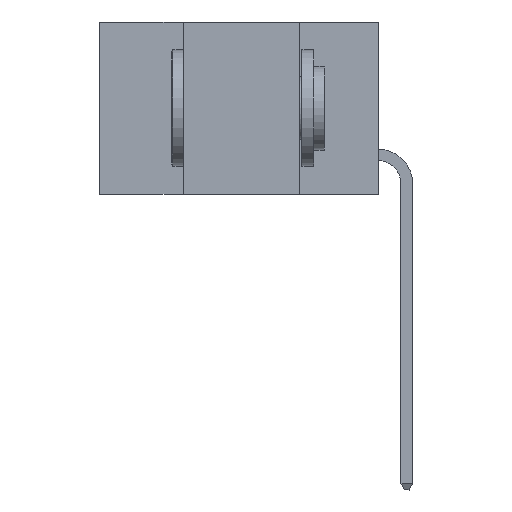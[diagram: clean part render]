
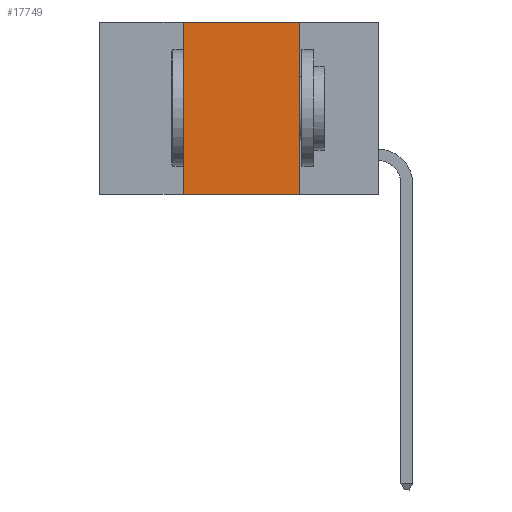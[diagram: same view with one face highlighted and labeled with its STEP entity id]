
A CAD part, left-side view. The second image highlights one B-rep face of the part: STEP entity #17749.
In plain terms, the highlighted planar face has unit normal (-1, 0, 0).
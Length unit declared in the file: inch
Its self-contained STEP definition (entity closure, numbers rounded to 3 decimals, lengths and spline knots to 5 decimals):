
#150 = CARTESIAN_POINT ( 'NONE',  ( 0., 0.42, 0. ) ) ;
#966 = VERTEX_POINT ( 'NONE', #23964 ) ;
#1774 = VERTEX_POINT ( 'NONE', #26614 ) ;
#4320 = CARTESIAN_POINT ( 'NONE',  ( 0., 0.17, 0. ) ) ;
#4855 = ORIENTED_EDGE ( 'NONE', *, *, #21750, .T. ) ;
#6186 = CARTESIAN_POINT ( 'NONE',  ( 0., 0.17, 0. ) ) ;
#7900 = DIRECTION ( 'NONE',  ( 0., -1., 0. ) ) ;
#9769 = EDGE_CURVE ( 'NONE', #966, #13858, #31250, .T. ) ;
#10986 = DIRECTION ( 'NONE',  ( 0., -1., 0. ) ) ;
#12270 = CARTESIAN_POINT ( 'NONE',  ( 0., 0.6, 0. ) ) ;
#12419 = VERTEX_POINT ( 'NONE', #4320 ) ;
#12866 = CARTESIAN_POINT ( 'NONE',  ( 0., 0.42, 0. ) ) ;
#12957 = DIRECTION ( 'NONE',  ( 0., 0., 1. ) ) ;
#13639 = VECTOR ( 'NONE', #27767, 39.37008 ) ;
#13858 = VERTEX_POINT ( 'NONE', #150 ) ;
#14344 = DIRECTION ( 'NONE',  ( 0., 0., -1. ) ) ;
#14470 = FACE_OUTER_BOUND ( 'NONE', #18750, .T. ) ;
#16296 = LINE ( 'NONE', #6186, #13639 ) ;
#16791 = ORIENTED_EDGE ( 'NONE', *, *, #18220, .F. ) ;
#17749 = ADVANCED_FACE ( 'NONE', ( #14470 ), #19234, .F. ) ;
#18220 = EDGE_CURVE ( 'NONE', #12419, #1774, #16296, .T. ) ;
#18742 = EDGE_CURVE ( 'NONE', #13858, #12419, #23878, .T. ) ;
#18750 = EDGE_LOOP ( 'NONE', ( #16791, #20926, #22518, #4855 ) ) ;
#19234 = PLANE ( 'NONE',  #23331 ) ;
#20926 = ORIENTED_EDGE ( 'NONE', *, *, #18742, .F. ) ;
#21750 = EDGE_CURVE ( 'NONE', #966, #1774, #28984, .T. ) ;
#21966 = VECTOR ( 'NONE', #10986, 39.37008 ) ;
#22518 = ORIENTED_EDGE ( 'NONE', *, *, #9769, .F. ) ;
#22539 = VECTOR ( 'NONE', #7900, 39.37008 ) ;
#23331 = AXIS2_PLACEMENT_3D ( 'NONE', #12270, #28849, #14344 ) ;
#23878 = LINE ( 'NONE', #30292, #21966 ) ;
#23964 = CARTESIAN_POINT ( 'NONE',  ( 0., 0.42, -0.37 ) ) ;
#26614 = CARTESIAN_POINT ( 'NONE',  ( 0., 0.17, -0.37 ) ) ;
#27669 = CARTESIAN_POINT ( 'NONE',  ( 0., 0.6, -0.37 ) ) ;
#27767 = DIRECTION ( 'NONE',  ( 0., 0., -1. ) ) ;
#27857 = VECTOR ( 'NONE', #12957, 39.37008 ) ;
#28849 = DIRECTION ( 'NONE',  ( 1., 0., 0. ) ) ;
#28984 = LINE ( 'NONE', #27669, #22539 ) ;
#30292 = CARTESIAN_POINT ( 'NONE',  ( 0., 0.6, 0. ) ) ;
#31250 = LINE ( 'NONE', #12866, #27857 ) ;
